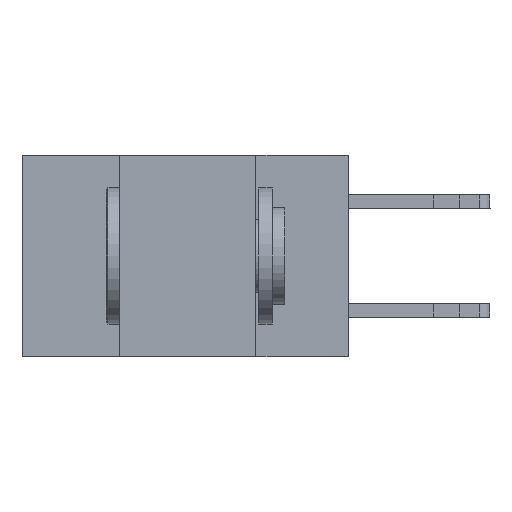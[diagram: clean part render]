
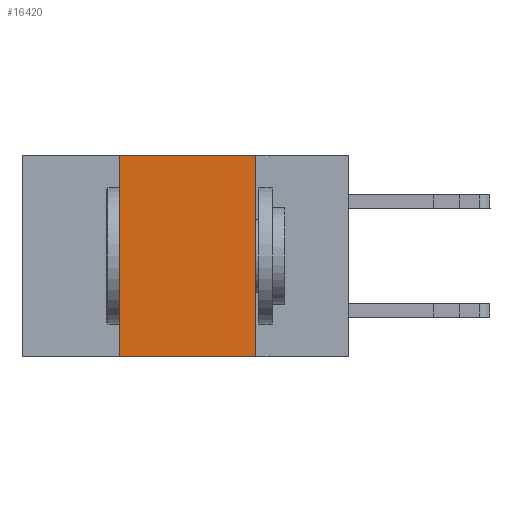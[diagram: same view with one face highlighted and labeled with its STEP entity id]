
A CAD part, left-side view. The second image highlights one B-rep face of the part: STEP entity #16420.
In plain terms, the highlighted planar face has unit normal (-1, 0, 0).
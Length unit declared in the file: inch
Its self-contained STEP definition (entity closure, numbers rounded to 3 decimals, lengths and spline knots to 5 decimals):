
#6 = ORIENTED_EDGE ( 'NONE', *, *, #13129, .F. ) ;
#827 = EDGE_CURVE ( 'NONE', #10149, #6108, #10787, .T. ) ;
#1354 = ORIENTED_EDGE ( 'NONE', *, *, #7719, .T. ) ;
#1700 = VECTOR ( 'NONE', #7077, 39.37008 ) ;
#1856 = CARTESIAN_POINT ( 'NONE',  ( 0., 0.42, -0.37 ) ) ;
#2207 = EDGE_LOOP ( 'NONE', ( #4852, #6, #5752, #1354 ) ) ;
#2342 = VECTOR ( 'NONE', #13157, 39.37008 ) ;
#3258 = LINE ( 'NONE', #3339, #8261 ) ;
#3339 = CARTESIAN_POINT ( 'NONE',  ( 0., 0.6, 0. ) ) ;
#3841 = DIRECTION ( 'NONE',  ( 1., 0., 0. ) ) ;
#4082 = CARTESIAN_POINT ( 'NONE',  ( 0., 0.42, 0. ) ) ;
#4200 = VERTEX_POINT ( 'NONE', #14216 ) ;
#4852 = ORIENTED_EDGE ( 'NONE', *, *, #12596, .F. ) ;
#5752 = ORIENTED_EDGE ( 'NONE', *, *, #827, .F. ) ;
#5942 = VECTOR ( 'NONE', #8478, 39.37008 ) ;
#6108 = VERTEX_POINT ( 'NONE', #4082 ) ;
#6183 = PLANE ( 'NONE',  #9171 ) ;
#7077 = DIRECTION ( 'NONE',  ( 0., -1., 0. ) ) ;
#7712 = FACE_OUTER_BOUND ( 'NONE', #2207, .T. ) ;
#7719 = EDGE_CURVE ( 'NONE', #10149, #12173, #11199, .T. ) ;
#7937 = CARTESIAN_POINT ( 'NONE',  ( 0., 0.17, -0.37 ) ) ;
#8261 = VECTOR ( 'NONE', #8505, 39.37008 ) ;
#8478 = DIRECTION ( 'NONE',  ( 0., 0., 1. ) ) ;
#8505 = DIRECTION ( 'NONE',  ( 0., -1., 0. ) ) ;
#8539 = CARTESIAN_POINT ( 'NONE',  ( 0., 0.6, -0.37 ) ) ;
#9171 = AXIS2_PLACEMENT_3D ( 'NONE', #16904, #3841, #13018 ) ;
#9230 = LINE ( 'NONE', #7937, #2342 ) ;
#10149 = VERTEX_POINT ( 'NONE', #13161 ) ;
#10787 = LINE ( 'NONE', #1856, #5942 ) ;
#11199 = LINE ( 'NONE', #8539, #1700 ) ;
#12173 = VERTEX_POINT ( 'NONE', #12778 ) ;
#12596 = EDGE_CURVE ( 'NONE', #4200, #12173, #9230, .T. ) ;
#12778 = CARTESIAN_POINT ( 'NONE',  ( 0., 0.17, -0.37 ) ) ;
#13018 = DIRECTION ( 'NONE',  ( 0., 0., -1. ) ) ;
#13129 = EDGE_CURVE ( 'NONE', #6108, #4200, #3258, .T. ) ;
#13157 = DIRECTION ( 'NONE',  ( 0., 0., -1. ) ) ;
#13161 = CARTESIAN_POINT ( 'NONE',  ( 0., 0.42, -0.37 ) ) ;
#14216 = CARTESIAN_POINT ( 'NONE',  ( 0., 0.17, 0. ) ) ;
#16420 = ADVANCED_FACE ( 'NONE', ( #7712 ), #6183, .F. ) ;
#16904 = CARTESIAN_POINT ( 'NONE',  ( 0., 0.6, 0. ) ) ;
